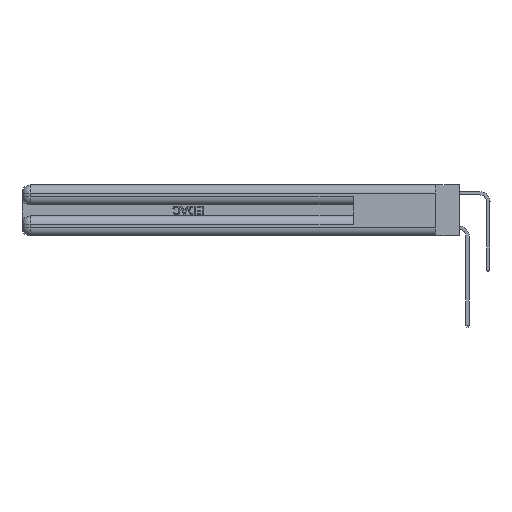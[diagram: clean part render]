
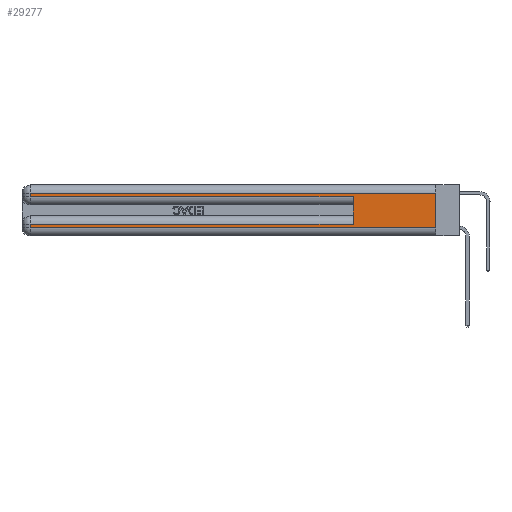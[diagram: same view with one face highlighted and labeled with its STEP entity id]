
A CAD part, left-side view. The second image highlights one B-rep face of the part: STEP entity #29277.
In plain terms, the highlighted planar face has unit normal (-1, 0, 0).
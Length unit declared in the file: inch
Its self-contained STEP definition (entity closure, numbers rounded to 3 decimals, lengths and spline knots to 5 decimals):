
#160 = CARTESIAN_POINT ( 'NONE',  ( 0., 0.6, 0.145 ) ) ;
#400 = CARTESIAN_POINT ( 'NONE',  ( 0., 2.94, 0.06 ) ) ;
#696 = CARTESIAN_POINT ( 'NONE',  ( 0., 0., 0.06 ) ) ;
#792 = CARTESIAN_POINT ( 'NONE',  ( 0., 0., 0.06 ) ) ;
#1155 = VERTEX_POINT ( 'NONE', #400 ) ;
#1295 = DIRECTION ( 'NONE',  ( 0., 0., -1. ) ) ;
#1625 = DIRECTION ( 'NONE',  ( 0., 1., 0. ) ) ;
#2572 = VERTEX_POINT ( 'NONE', #26774 ) ;
#2737 = FACE_OUTER_BOUND ( 'NONE', #5122, .T. ) ;
#3432 = ORIENTED_EDGE ( 'NONE', *, *, #23886, .T. ) ;
#3890 = CARTESIAN_POINT ( 'NONE',  ( 0., 0., 0.37 ) ) ;
#4160 = VERTEX_POINT ( 'NONE', #18620 ) ;
#4177 = VECTOR ( 'NONE', #11763, 39.37008 ) ;
#4557 = ORIENTED_EDGE ( 'NONE', *, *, #13549, .T. ) ;
#4669 = CARTESIAN_POINT ( 'NONE',  ( 0., 2.94, 0.37 ) ) ;
#5042 = LINE ( 'NONE', #11647, #21693 ) ;
#5045 = VECTOR ( 'NONE', #21963, 39.37008 ) ;
#5122 = EDGE_LOOP ( 'NONE', ( #20448, #4557, #8946, #17418, #9537, #3432, #20196, #33046 ) ) ;
#6557 = PLANE ( 'NONE',  #25615 ) ;
#7160 = LINE ( 'NONE', #696, #5045 ) ;
#8316 = DIRECTION ( 'NONE',  ( 0., 1., 0. ) ) ;
#8946 = ORIENTED_EDGE ( 'NONE', *, *, #26042, .T. ) ;
#9370 = CARTESIAN_POINT ( 'NONE',  ( 0., 0.6, 0.085 ) ) ;
#9537 = ORIENTED_EDGE ( 'NONE', *, *, #34054, .F. ) ;
#9721 = VERTEX_POINT ( 'NONE', #9370 ) ;
#11048 = VERTEX_POINT ( 'NONE', #15891 ) ;
#11647 = CARTESIAN_POINT ( 'NONE',  ( 0., 0., 0.285 ) ) ;
#11763 = DIRECTION ( 'NONE',  ( 0., 0., 1. ) ) ;
#12375 = VECTOR ( 'NONE', #1295, 39.37008 ) ;
#12569 = LINE ( 'NONE', #160, #4177 ) ;
#13009 = EDGE_CURVE ( 'NONE', #18244, #4160, #5042, .T. ) ;
#13160 = CARTESIAN_POINT ( 'NONE',  ( 0., 2.94, 0.31 ) ) ;
#13549 = EDGE_CURVE ( 'NONE', #11048, #17247, #31696, .T. ) ;
#14777 = CARTESIAN_POINT ( 'NONE',  ( 0., 2.94, 0.37 ) ) ;
#15891 = CARTESIAN_POINT ( 'NONE',  ( 0., 0., 0.31 ) ) ;
#17247 = VERTEX_POINT ( 'NONE', #13160 ) ;
#17418 = ORIENTED_EDGE ( 'NONE', *, *, #13009, .T. ) ;
#17808 = DIRECTION ( 'NONE',  ( 0., 0., -1. ) ) ;
#18191 = EDGE_CURVE ( 'NONE', #11048, #18470, #19445, .T. ) ;
#18244 = VERTEX_POINT ( 'NONE', #30527 ) ;
#18470 = VERTEX_POINT ( 'NONE', #792 ) ;
#18620 = CARTESIAN_POINT ( 'NONE',  ( 0., 0.6, 0.285 ) ) ;
#19445 = LINE ( 'NONE', #3890, #12375 ) ;
#19947 = CARTESIAN_POINT ( 'NONE',  ( 0., 0., 0.37 ) ) ;
#20061 = DIRECTION ( 'NONE',  ( 0., 0., -1. ) ) ;
#20196 = ORIENTED_EDGE ( 'NONE', *, *, #28064, .T. ) ;
#20448 = ORIENTED_EDGE ( 'NONE', *, *, #18191, .F. ) ;
#21693 = VECTOR ( 'NONE', #32964, 39.37008 ) ;
#21963 = DIRECTION ( 'NONE',  ( 0., -1., 0. ) ) ;
#22378 = EDGE_CURVE ( 'NONE', #1155, #18470, #7160, .T. ) ;
#22885 = CARTESIAN_POINT ( 'NONE',  ( 0., 0., 0.31 ) ) ;
#23325 = LINE ( 'NONE', #29581, #34140 ) ;
#23362 = DIRECTION ( 'NONE',  ( 0., 0., -1. ) ) ;
#23886 = EDGE_CURVE ( 'NONE', #9721, #2572, #23325, .T. ) ;
#25441 = VECTOR ( 'NONE', #1625, 39.37008 ) ;
#25615 = AXIS2_PLACEMENT_3D ( 'NONE', #19947, #27691, #20061 ) ;
#26042 = EDGE_CURVE ( 'NONE', #17247, #18244, #34255, .T. ) ;
#26774 = CARTESIAN_POINT ( 'NONE',  ( 0., 2.94, 0.085 ) ) ;
#27032 = VECTOR ( 'NONE', #17808, 39.37008 ) ;
#27470 = LINE ( 'NONE', #14777, #27032 ) ;
#27691 = DIRECTION ( 'NONE',  ( 1., 0., 0. ) ) ;
#28064 = EDGE_CURVE ( 'NONE', #2572, #1155, #27470, .T. ) ;
#29277 = ADVANCED_FACE ( 'NONE', ( #2737 ), #6557, .F. ) ;
#29581 = CARTESIAN_POINT ( 'NONE',  ( 0., 0., 0.085 ) ) ;
#30527 = CARTESIAN_POINT ( 'NONE',  ( 0., 2.94, 0.285 ) ) ;
#30945 = VECTOR ( 'NONE', #23362, 39.37008 ) ;
#31696 = LINE ( 'NONE', #22885, #25441 ) ;
#32964 = DIRECTION ( 'NONE',  ( 0., -1., 0. ) ) ;
#33046 = ORIENTED_EDGE ( 'NONE', *, *, #22378, .T. ) ;
#34054 = EDGE_CURVE ( 'NONE', #9721, #4160, #12569, .T. ) ;
#34140 = VECTOR ( 'NONE', #8316, 39.37008 ) ;
#34255 = LINE ( 'NONE', #4669, #30945 ) ;
